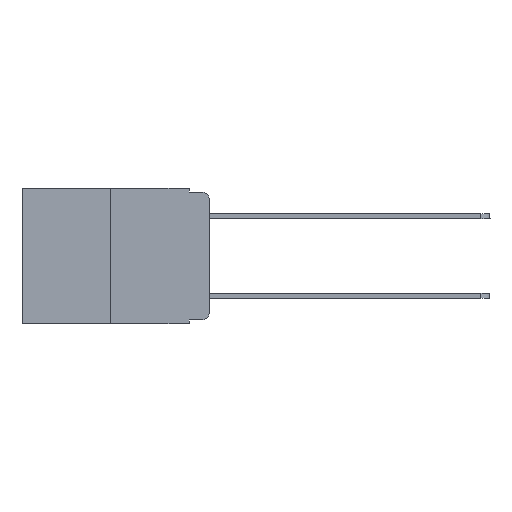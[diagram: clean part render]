
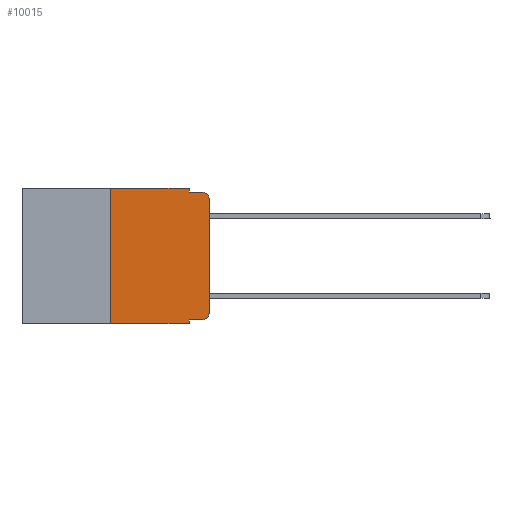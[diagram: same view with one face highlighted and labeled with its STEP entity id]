
A CAD part, left-side view. The second image highlights one B-rep face of the part: STEP entity #10015.
In plain terms, the highlighted planar face has unit normal (-1, 0, 0).
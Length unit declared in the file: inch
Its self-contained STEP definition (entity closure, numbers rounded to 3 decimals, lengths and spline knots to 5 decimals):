
#431 = DIRECTION ( 'NONE',  ( 0., 0., -1. ) ) ;
#471 = DIRECTION ( 'NONE',  ( -1., 0., 0. ) ) ;
#802 = ORIENTED_EDGE ( 'NONE', *, *, #7535, .F. ) ;
#1008 = DIRECTION ( 'NONE',  ( -1., 0., 0. ) ) ;
#1595 = VECTOR ( 'NONE', #9724, 39.37008 ) ;
#2834 = VECTOR ( 'NONE', #21974, 39.37008 ) ;
#2996 = CARTESIAN_POINT ( 'NONE',  ( 0., 0.051, -0.01 ) ) ;
#3656 = ORIENTED_EDGE ( 'NONE', *, *, #18128, .F. ) ;
#3705 = CIRCLE ( 'NONE', #7297, 0.02 ) ;
#3815 = CARTESIAN_POINT ( 'NONE',  ( 0., 0.051, -0.333 ) ) ;
#4576 = CARTESIAN_POINT ( 'NONE',  ( 0., 0.02, -0.313 ) ) ;
#4703 = VERTEX_POINT ( 'NONE', #20580 ) ;
#4932 = LINE ( 'NONE', #16009, #2834 ) ;
#5032 = CARTESIAN_POINT ( 'NONE',  ( 0., 0.02, -0.03 ) ) ;
#5217 = ORIENTED_EDGE ( 'NONE', *, *, #13439, .F. ) ;
#5613 = LINE ( 'NONE', #19368, #15509 ) ;
#5752 = CARTESIAN_POINT ( 'NONE',  ( 0., 0.051, -0.333 ) ) ;
#5825 = LINE ( 'NONE', #16197, #19252 ) ;
#6218 = CARTESIAN_POINT ( 'NONE',  ( 0., 0.25, -0.343 ) ) ;
#6700 = LINE ( 'NONE', #5752, #1595 ) ;
#6905 = CARTESIAN_POINT ( 'NONE',  ( 0., 0.02, -0.01 ) ) ;
#6924 = DIRECTION ( 'NONE',  ( 0., 0., -1. ) ) ;
#7025 = VERTEX_POINT ( 'NONE', #15662 ) ;
#7048 = AXIS2_PLACEMENT_3D ( 'NONE', #4576, #471, #15855 ) ;
#7133 = CARTESIAN_POINT ( 'NONE',  ( 0., 0.473, -0.343 ) ) ;
#7262 = VECTOR ( 'NONE', #18429, 39.37008 ) ;
#7297 = AXIS2_PLACEMENT_3D ( 'NONE', #5032, #1008, #18367 ) ;
#7329 = ORIENTED_EDGE ( 'NONE', *, *, #15493, .T. ) ;
#7535 = EDGE_CURVE ( 'NONE', #4703, #8524, #5825, .T. ) ;
#8167 = CARTESIAN_POINT ( 'NONE',  ( 0., 0.051, -0.01 ) ) ;
#8216 = ORIENTED_EDGE ( 'NONE', *, *, #14940, .F. ) ;
#8524 = VERTEX_POINT ( 'NONE', #8167 ) ;
#9069 = CARTESIAN_POINT ( 'NONE',  ( 0., 0., -0.313 ) ) ;
#9525 = ORIENTED_EDGE ( 'NONE', *, *, #18332, .T. ) ;
#9724 = DIRECTION ( 'NONE',  ( 0., -1., 0. ) ) ;
#9993 = LINE ( 'NONE', #16511, #7262 ) ;
#10015 = ADVANCED_FACE ( 'NONE', ( #12736 ), #17785, .F. ) ;
#10157 = EDGE_CURVE ( 'NONE', #7025, #19202, #3705, .T. ) ;
#10164 = LINE ( 'NONE', #2996, #17592 ) ;
#10315 = DIRECTION ( 'NONE',  ( 0., 0., -1. ) ) ;
#10356 = AXIS2_PLACEMENT_3D ( 'NONE', #21601, #21693, #10315 ) ;
#11012 = ORIENTED_EDGE ( 'NONE', *, *, #18526, .T. ) ;
#11163 = DIRECTION ( 'NONE',  ( 0., -1., 0. ) ) ;
#12736 = FACE_OUTER_BOUND ( 'NONE', #16930, .T. ) ;
#12752 = ORIENTED_EDGE ( 'NONE', *, *, #10157, .T. ) ;
#13439 = EDGE_CURVE ( 'NONE', #14603, #19017, #5613, .T. ) ;
#14221 = DIRECTION ( 'NONE',  ( 0., -1., 0. ) ) ;
#14603 = VERTEX_POINT ( 'NONE', #3815 ) ;
#14940 = EDGE_CURVE ( 'NONE', #21090, #21829, #4932, .T. ) ;
#15493 = EDGE_CURVE ( 'NONE', #14603, #24319, #6700, .T. ) ;
#15509 = VECTOR ( 'NONE', #431, 39.37008 ) ;
#15662 = CARTESIAN_POINT ( 'NONE',  ( 0., 0., -0.03 ) ) ;
#15774 = CARTESIAN_POINT ( 'NONE',  ( 0., 0.051, -0.343 ) ) ;
#15796 = LINE ( 'NONE', #7133, #20231 ) ;
#15849 = EDGE_CURVE ( 'NONE', #21829, #4703, #9993, .T. ) ;
#15855 = DIRECTION ( 'NONE',  ( 0., 0., -1. ) ) ;
#16009 = CARTESIAN_POINT ( 'NONE',  ( 0., 0.25, 0. ) ) ;
#16197 = CARTESIAN_POINT ( 'NONE',  ( 0., 0.051, 0. ) ) ;
#16455 = ORIENTED_EDGE ( 'NONE', *, *, #23856, .T. ) ;
#16511 = CARTESIAN_POINT ( 'NONE',  ( 0., 0.473, 0. ) ) ;
#16930 = EDGE_LOOP ( 'NONE', ( #11012, #12752, #3656, #802, #21281, #8216, #9525, #5217, #7329, #16455 ) ) ;
#16942 = CARTESIAN_POINT ( 'NONE',  ( 0., 0.25, 0. ) ) ;
#16984 = VECTOR ( 'NONE', #19336, 39.37008 ) ;
#17592 = VECTOR ( 'NONE', #14221, 39.37008 ) ;
#17687 = CIRCLE ( 'NONE', #7048, 0.02 ) ;
#17785 = PLANE ( 'NONE',  #10356 ) ;
#18128 = EDGE_CURVE ( 'NONE', #8524, #19202, #10164, .T. ) ;
#18332 = EDGE_CURVE ( 'NONE', #21090, #19017, #15796, .T. ) ;
#18367 = DIRECTION ( 'NONE',  ( 0., 0., -1. ) ) ;
#18429 = DIRECTION ( 'NONE',  ( 0., -1., 0. ) ) ;
#18526 = EDGE_CURVE ( 'NONE', #23001, #7025, #24432, .T. ) ;
#19017 = VERTEX_POINT ( 'NONE', #15774 ) ;
#19202 = VERTEX_POINT ( 'NONE', #6905 ) ;
#19252 = VECTOR ( 'NONE', #6924, 39.37008 ) ;
#19336 = DIRECTION ( 'NONE',  ( 0., 0., 1. ) ) ;
#19368 = CARTESIAN_POINT ( 'NONE',  ( 0., 0.051, 0. ) ) ;
#19411 = CARTESIAN_POINT ( 'NONE',  ( 0., 0., 0. ) ) ;
#20231 = VECTOR ( 'NONE', #11163, 39.37008 ) ;
#20580 = CARTESIAN_POINT ( 'NONE',  ( 0., 0.051, 0. ) ) ;
#21090 = VERTEX_POINT ( 'NONE', #6218 ) ;
#21281 = ORIENTED_EDGE ( 'NONE', *, *, #15849, .F. ) ;
#21601 = CARTESIAN_POINT ( 'NONE',  ( 0., 0.473, 0. ) ) ;
#21693 = DIRECTION ( 'NONE',  ( 1., 0., 0. ) ) ;
#21829 = VERTEX_POINT ( 'NONE', #16942 ) ;
#21974 = DIRECTION ( 'NONE',  ( 0., 0., 1. ) ) ;
#22796 = CARTESIAN_POINT ( 'NONE',  ( 0., 0.02, -0.333 ) ) ;
#23001 = VERTEX_POINT ( 'NONE', #9069 ) ;
#23856 = EDGE_CURVE ( 'NONE', #24319, #23001, #17687, .T. ) ;
#24319 = VERTEX_POINT ( 'NONE', #22796 ) ;
#24432 = LINE ( 'NONE', #19411, #16984 ) ;
